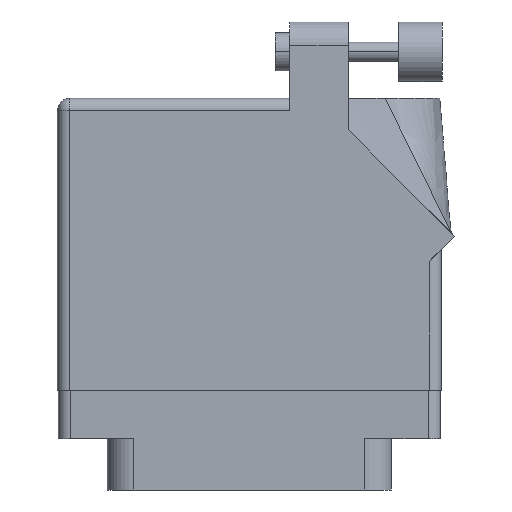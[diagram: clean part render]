
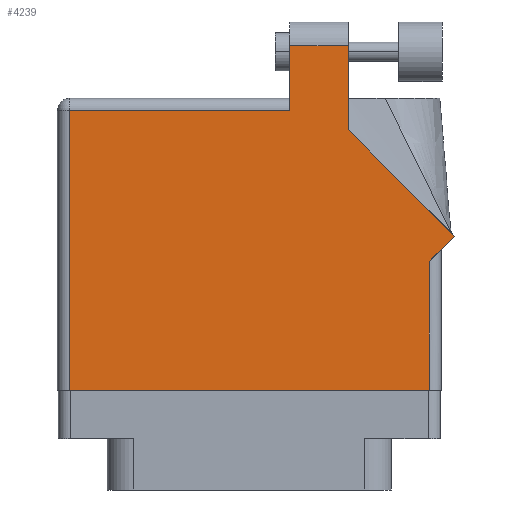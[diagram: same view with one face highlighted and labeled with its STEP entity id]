
A CAD part, front view. The second image highlights one B-rep face of the part: STEP entity #4239.
In plain terms, the highlighted face is planar.
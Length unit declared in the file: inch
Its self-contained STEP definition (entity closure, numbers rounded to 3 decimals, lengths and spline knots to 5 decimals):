
#382 = CARTESIAN_POINT ( 'NONE',  ( 0.212, 1.43, 0.455 ) ) ;
#744 = VECTOR ( 'NONE', #25239, 39.37008 ) ;
#1257 = DIRECTION ( 'NONE',  ( 0., 1., 0. ) ) ;
#1523 = LINE ( 'NONE', #33083, #16859 ) ;
#1769 = CARTESIAN_POINT ( 'NONE',  ( 0.519, 1.26442, 0.455 ) ) ;
#2228 = CARTESIAN_POINT ( 'NONE',  ( 0.943, -0.1, 0.455 ) ) ;
#2646 = ORIENTED_EDGE ( 'NONE', *, *, #14900, .T. ) ;
#3636 = VECTOR ( 'NONE', #28397, 39.37008 ) ;
#4239 = ADVANCED_FACE ( 'NONE', ( #4877 ), #23026, .F. ) ;
#4299 = VECTOR ( 'NONE', #39024, 39.37008 ) ;
#4402 = EDGE_CURVE ( 'NONE', #38469, #18130, #1523, .T. ) ;
#4778 = VERTEX_POINT ( 'NONE', #20225 ) ;
#4877 = FACE_OUTER_BOUND ( 'NONE', #15979, .T. ) ;
#6041 = LINE ( 'NONE', #18621, #3636 ) ;
#6117 = LINE ( 'NONE', #9623, #31253 ) ;
#6696 = ORIENTED_EDGE ( 'NONE', *, *, #4402, .T. ) ;
#6955 = VERTEX_POINT ( 'NONE', #2228 ) ;
#7651 = DIRECTION ( 'NONE',  ( -1., 0., 0. ) ) ;
#8377 = CARTESIAN_POINT ( 'NONE',  ( 1.07571, 0.70771, 0.455 ) ) ;
#9548 = EDGE_CURVE ( 'NONE', #27899, #6955, #18034, .T. ) ;
#9623 = CARTESIAN_POINT ( 'NONE',  ( -1.005, 1.368, 0.455 ) ) ;
#10214 = VECTOR ( 'NONE', #34928, 39.37008 ) ;
#10574 = VERTEX_POINT ( 'NONE', #11078 ) ;
#11078 = CARTESIAN_POINT ( 'NONE',  ( 0.943, 0.575, 0.455 ) ) ;
#11935 = ORIENTED_EDGE ( 'NONE', *, *, #13077, .T. ) ;
#12066 = EDGE_CURVE ( 'NONE', #18130, #4778, #12641, .T. ) ;
#12641 = LINE ( 'NONE', #382, #10214 ) ;
#13048 = VERTEX_POINT ( 'NONE', #22256 ) ;
#13054 = CARTESIAN_POINT ( 'NONE',  ( -1.005, -0.1, 0.455 ) ) ;
#13077 = EDGE_CURVE ( 'NONE', #13048, #38469, #15955, .T. ) ;
#13383 = CARTESIAN_POINT ( 'NONE',  ( 1.07571, 0.70771, 0.455 ) ) ;
#13762 = VERTEX_POINT ( 'NONE', #13383 ) ;
#14900 = EDGE_CURVE ( 'NONE', #13762, #13048, #27002, .T. ) ;
#15955 = LINE ( 'NONE', #1769, #27071 ) ;
#15979 = EDGE_LOOP ( 'NONE', ( #11935, #6696, #38995, #16127, #18774, #22201, #19767, #16281, #2646 ) ) ;
#16127 = ORIENTED_EDGE ( 'NONE', *, *, #16643, .T. ) ;
#16281 = ORIENTED_EDGE ( 'NONE', *, *, #24258, .T. ) ;
#16643 = EDGE_CURVE ( 'NONE', #4778, #25416, #6117, .T. ) ;
#16859 = VECTOR ( 'NONE', #17842, 39.37008 ) ;
#17842 = DIRECTION ( 'NONE',  ( -1., 0., 0. ) ) ;
#18034 = LINE ( 'NONE', #13054, #744 ) ;
#18130 = VERTEX_POINT ( 'NONE', #19165 ) ;
#18536 = VECTOR ( 'NONE', #24898, 39.37008 ) ;
#18621 = CARTESIAN_POINT ( 'NONE',  ( 1.005, 0.637, 0.455 ) ) ;
#18774 = ORIENTED_EDGE ( 'NONE', *, *, #29520, .T. ) ;
#19165 = CARTESIAN_POINT ( 'NONE',  ( 0.212, 1.705, 0.455 ) ) ;
#19767 = ORIENTED_EDGE ( 'NONE', *, *, #35394, .T. ) ;
#20225 = CARTESIAN_POINT ( 'NONE',  ( 0.212, 1.368, 0.455 ) ) ;
#22201 = ORIENTED_EDGE ( 'NONE', *, *, #9548, .T. ) ;
#22256 = CARTESIAN_POINT ( 'NONE',  ( 0.519, 1.26442, 0.455 ) ) ;
#23026 = PLANE ( 'NONE',  #29290 ) ;
#23410 = LINE ( 'NONE', #27998, #18536 ) ;
#24258 = EDGE_CURVE ( 'NONE', #10574, #13762, #6041, .T. ) ;
#24898 = DIRECTION ( 'NONE',  ( 0., -1., 0. ) ) ;
#24964 = VECTOR ( 'NONE', #1257, 39.37008 ) ;
#25239 = DIRECTION ( 'NONE',  ( 1., 0., 0. ) ) ;
#25416 = VERTEX_POINT ( 'NONE', #27691 ) ;
#26426 = CARTESIAN_POINT ( 'NONE',  ( -1.005, 1.43, 0.455 ) ) ;
#27002 = LINE ( 'NONE', #8377, #4299 ) ;
#27071 = VECTOR ( 'NONE', #29317, 39.37008 ) ;
#27691 = CARTESIAN_POINT ( 'NONE',  ( -0.943, 1.368, 0.455 ) ) ;
#27899 = VERTEX_POINT ( 'NONE', #38631 ) ;
#27998 = CARTESIAN_POINT ( 'NONE',  ( -0.943, -0.1, 0.455 ) ) ;
#28397 = DIRECTION ( 'NONE',  ( 0.707, 0.707, 0. ) ) ;
#28526 = CARTESIAN_POINT ( 'NONE',  ( 0.943, 0.637, 0.455 ) ) ;
#29290 = AXIS2_PLACEMENT_3D ( 'NONE', #26426, #32537, #7651 ) ;
#29317 = DIRECTION ( 'NONE',  ( 0., 1., 0. ) ) ;
#29520 = EDGE_CURVE ( 'NONE', #25416, #27899, #23410, .T. ) ;
#30052 = CARTESIAN_POINT ( 'NONE',  ( 0.519, 1.705, 0.455 ) ) ;
#30911 = DIRECTION ( 'NONE',  ( -1., 0., 0. ) ) ;
#31253 = VECTOR ( 'NONE', #30911, 39.37008 ) ;
#32215 = LINE ( 'NONE', #28526, #24964 ) ;
#32537 = DIRECTION ( 'NONE',  ( 0., 0., -1. ) ) ;
#33083 = CARTESIAN_POINT ( 'NONE',  ( 0.212, 1.705, 0.455 ) ) ;
#34928 = DIRECTION ( 'NONE',  ( 0., -1., 0. ) ) ;
#35394 = EDGE_CURVE ( 'NONE', #6955, #10574, #32215, .T. ) ;
#38469 = VERTEX_POINT ( 'NONE', #30052 ) ;
#38631 = CARTESIAN_POINT ( 'NONE',  ( -0.943, -0.1, 0.455 ) ) ;
#38995 = ORIENTED_EDGE ( 'NONE', *, *, #12066, .T. ) ;
#39024 = DIRECTION ( 'NONE',  ( -0.707, 0.707, 0. ) ) ;
